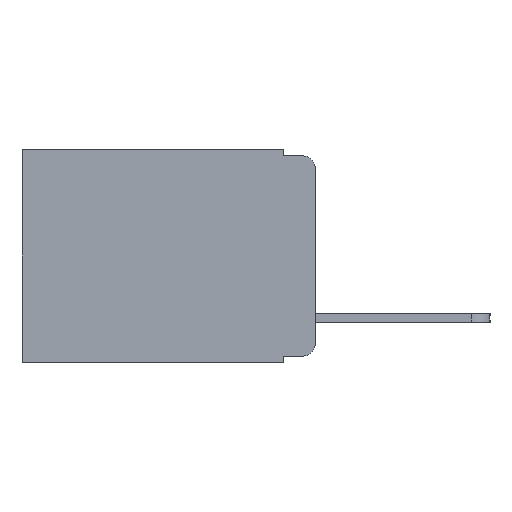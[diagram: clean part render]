
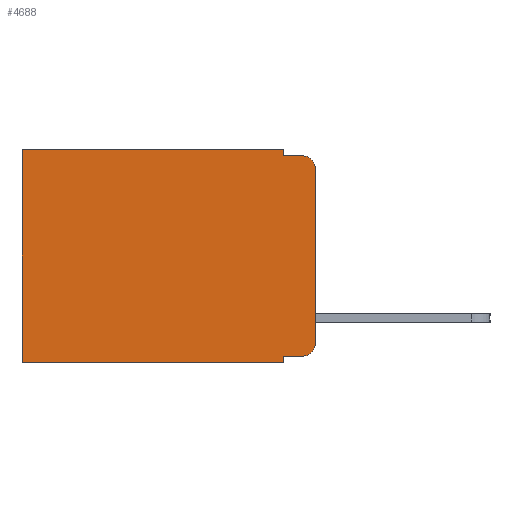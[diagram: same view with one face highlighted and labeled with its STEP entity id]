
A CAD part, left-side view. The second image highlights one B-rep face of the part: STEP entity #4688.
In plain terms, the highlighted planar face has unit normal (-1, 0, 0).
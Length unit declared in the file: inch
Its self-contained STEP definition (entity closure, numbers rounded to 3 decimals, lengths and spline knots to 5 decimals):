
#60 = LINE ( 'NONE', #9399, #8665 ) ;
#61 = CARTESIAN_POINT ( 'NONE',  ( 0.298, 0., -0.03 ) ) ;
#112 = VERTEX_POINT ( 'NONE', #10145 ) ;
#656 = VERTEX_POINT ( 'NONE', #8164 ) ;
#770 = VERTEX_POINT ( 'NONE', #9275 ) ;
#1095 = VECTOR ( 'NONE', #1578, 39.37008 ) ;
#1219 = VECTOR ( 'NONE', #2417, 39.37008 ) ;
#1226 = DIRECTION ( 'NONE',  ( 0., -1., 0. ) ) ;
#1516 = LINE ( 'NONE', #10871, #1219 ) ;
#1549 = CARTESIAN_POINT ( 'NONE',  ( 0.298, 0.051, 0. ) ) ;
#1578 = DIRECTION ( 'NONE',  ( 0., 0., -1. ) ) ;
#1817 = VERTEX_POINT ( 'NONE', #61 ) ;
#1896 = VERTEX_POINT ( 'NONE', #8033 ) ;
#2393 = VERTEX_POINT ( 'NONE', #5378 ) ;
#2417 = DIRECTION ( 'NONE',  ( 0., 1., 0. ) ) ;
#2497 = VERTEX_POINT ( 'NONE', #10774 ) ;
#2641 = CARTESIAN_POINT ( 'NONE',  ( 0.298, 0.473, -0.343 ) ) ;
#2788 = EDGE_CURVE ( 'NONE', #9426, #770, #9728, .T. ) ;
#3360 = VECTOR ( 'NONE', #9201, 39.37008 ) ;
#3573 = ORIENTED_EDGE ( 'NONE', *, *, #3994, .T. ) ;
#3612 = EDGE_CURVE ( 'NONE', #1817, #656, #6868, .T. ) ;
#3930 = FACE_OUTER_BOUND ( 'NONE', #5710, .T. ) ;
#3994 = EDGE_CURVE ( 'NONE', #1817, #770, #7665, .T. ) ;
#4277 = PLANE ( 'NONE',  #6278 ) ;
#4461 = ORIENTED_EDGE ( 'NONE', *, *, #5916, .T. ) ;
#4585 = DIRECTION ( 'NONE',  ( 0., 0., -1. ) ) ;
#4688 = ADVANCED_FACE ( 'NONE', ( #3930 ), #4277, .F. ) ;
#4719 = EDGE_CURVE ( 'NONE', #9778, #5798, #10119, .T. ) ;
#5005 = ORIENTED_EDGE ( 'NONE', *, *, #5341, .T. ) ;
#5010 = LINE ( 'NONE', #10709, #8012 ) ;
#5142 = DIRECTION ( 'NONE',  ( 0., 0., -1. ) ) ;
#5341 = EDGE_CURVE ( 'NONE', #2497, #656, #10481, .T. ) ;
#5358 = DIRECTION ( 'NONE',  ( 0., -1., 0. ) ) ;
#5378 = CARTESIAN_POINT ( 'NONE',  ( 0.298, 0.473, 0. ) ) ;
#5417 = LINE ( 'NONE', #8276, #9561 ) ;
#5710 = EDGE_LOOP ( 'NONE', ( #9838, #3573, #9647, #10070, #9944, #9876, #9618, #8305, #4461, #5005 ) ) ;
#5798 = VERTEX_POINT ( 'NONE', #2641 ) ;
#5916 = EDGE_CURVE ( 'NONE', #1896, #2497, #5010, .T. ) ;
#6034 = CARTESIAN_POINT ( 'NONE',  ( 0.298, 0., 0. ) ) ;
#6278 = AXIS2_PLACEMENT_3D ( 'NONE', #6034, #7826, #7771 ) ;
#6868 = LINE ( 'NONE', #10716, #7400 ) ;
#6993 = AXIS2_PLACEMENT_3D ( 'NONE', #9071, #9866, #10137 ) ;
#7049 = EDGE_CURVE ( 'NONE', #1896, #9778, #10317, .T. ) ;
#7400 = VECTOR ( 'NONE', #4585, 39.37008 ) ;
#7627 = EDGE_CURVE ( 'NONE', #2393, #5798, #60, .T. ) ;
#7665 = CIRCLE ( 'NONE', #10026, 0.02 ) ;
#7737 = DIRECTION ( 'NONE',  ( -1., 0., 0. ) ) ;
#7771 = DIRECTION ( 'NONE',  ( 0., 0., -1. ) ) ;
#7822 = VECTOR ( 'NONE', #5358, 39.37008 ) ;
#7826 = DIRECTION ( 'NONE',  ( 1., 0., 0. ) ) ;
#7928 = CARTESIAN_POINT ( 'NONE',  ( 0.298, 0.051, -0.343 ) ) ;
#7979 = CARTESIAN_POINT ( 'NONE',  ( 0.298, 0.051, -0.01 ) ) ;
#8012 = VECTOR ( 'NONE', #1226, 39.37008 ) ;
#8033 = CARTESIAN_POINT ( 'NONE',  ( 0.298, 0.051, -0.333 ) ) ;
#8164 = CARTESIAN_POINT ( 'NONE',  ( 0.298, 0., -0.313 ) ) ;
#8174 = EDGE_CURVE ( 'NONE', #112, #2393, #1516, .T. ) ;
#8276 = CARTESIAN_POINT ( 'NONE',  ( 0.298, 0.051, 0. ) ) ;
#8305 = ORIENTED_EDGE ( 'NONE', *, *, #7049, .F. ) ;
#8656 = DIRECTION ( 'NONE',  ( 0., 0., -1. ) ) ;
#8665 = VECTOR ( 'NONE', #8656, 39.37008 ) ;
#8931 = CARTESIAN_POINT ( 'NONE',  ( 0.298, 0., -0.343 ) ) ;
#9071 = CARTESIAN_POINT ( 'NONE',  ( 0.298, 0.02, -0.313 ) ) ;
#9201 = DIRECTION ( 'NONE',  ( 0., 1., 0. ) ) ;
#9275 = CARTESIAN_POINT ( 'NONE',  ( 0.298, 0.02, -0.01 ) ) ;
#9399 = CARTESIAN_POINT ( 'NONE',  ( 0.298, 0.473, 0. ) ) ;
#9426 = VERTEX_POINT ( 'NONE', #10747 ) ;
#9561 = VECTOR ( 'NONE', #10764, 39.37008 ) ;
#9618 = ORIENTED_EDGE ( 'NONE', *, *, #4719, .F. ) ;
#9647 = ORIENTED_EDGE ( 'NONE', *, *, #2788, .F. ) ;
#9728 = LINE ( 'NONE', #7979, #7822 ) ;
#9778 = VERTEX_POINT ( 'NONE', #7928 ) ;
#9838 = ORIENTED_EDGE ( 'NONE', *, *, #3612, .F. ) ;
#9866 = DIRECTION ( 'NONE',  ( -1., 0., 0. ) ) ;
#9876 = ORIENTED_EDGE ( 'NONE', *, *, #7627, .T. ) ;
#9944 = ORIENTED_EDGE ( 'NONE', *, *, #8174, .T. ) ;
#10026 = AXIS2_PLACEMENT_3D ( 'NONE', #10091, #7737, #5142 ) ;
#10070 = ORIENTED_EDGE ( 'NONE', *, *, #10395, .F. ) ;
#10091 = CARTESIAN_POINT ( 'NONE',  ( 0.298, 0.02, -0.03 ) ) ;
#10119 = LINE ( 'NONE', #8931, #3360 ) ;
#10137 = DIRECTION ( 'NONE',  ( 0., 0., -1. ) ) ;
#10145 = CARTESIAN_POINT ( 'NONE',  ( 0.298, 0.051, 0. ) ) ;
#10317 = LINE ( 'NONE', #1549, #1095 ) ;
#10395 = EDGE_CURVE ( 'NONE', #112, #9426, #5417, .T. ) ;
#10481 = CIRCLE ( 'NONE', #6993, 0.02 ) ;
#10709 = CARTESIAN_POINT ( 'NONE',  ( 0.298, 0.051, -0.333 ) ) ;
#10716 = CARTESIAN_POINT ( 'NONE',  ( 0.298, 0., 0. ) ) ;
#10747 = CARTESIAN_POINT ( 'NONE',  ( 0.298, 0.051, -0.01 ) ) ;
#10764 = DIRECTION ( 'NONE',  ( 0., 0., -1. ) ) ;
#10774 = CARTESIAN_POINT ( 'NONE',  ( 0.298, 0.02, -0.333 ) ) ;
#10871 = CARTESIAN_POINT ( 'NONE',  ( 0.298, 0., 0. ) ) ;
